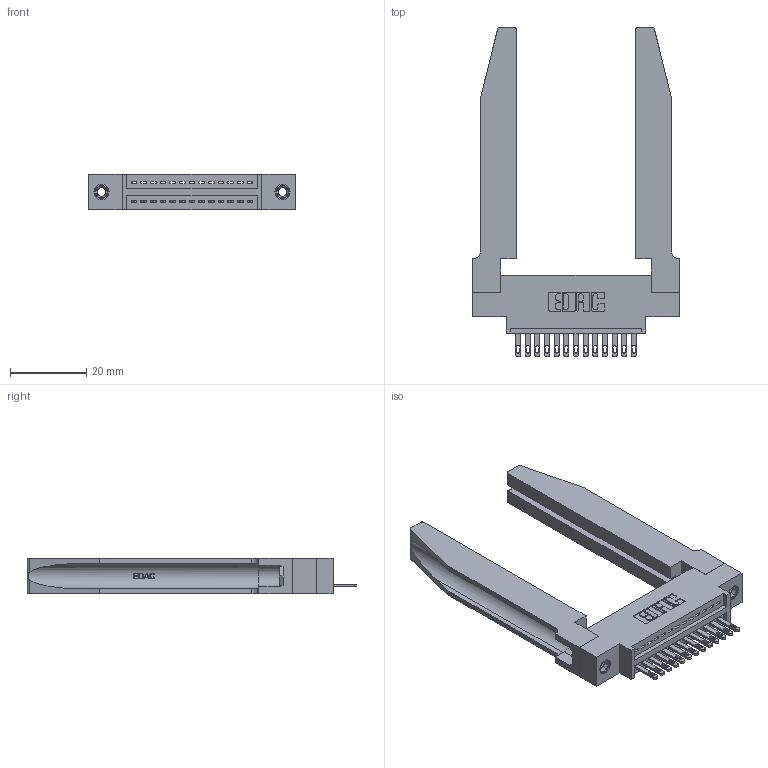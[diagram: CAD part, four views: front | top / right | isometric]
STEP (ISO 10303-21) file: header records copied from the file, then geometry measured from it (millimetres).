
FILE_DESCRIPTION (( 'STEP AP203' ), '1' );
FILE_NAME ('345-013-500-678.STEP', '2019-10-04T02:57:16', ( '' ), ( '' ), 'SwSTEP 2.0', 'SolidWorks 2016', '' );
FILE_SCHEMA (( 'CONFIG_CONTROL_DESIGN' ));
Length unit declared in the file: inch
Products named in the file (5): 345-292-001_345-293-100; 345-250-001_345-250-001-102; 345-220-078_345-220-078; 345 Part_0.170 Offset - 0.156 Dia-TH; 345-013-500-678
Assembly tree (18 placements, depth 2):
  345-013-500-678
    345 Part_0.170 Offset - 0.156 Dia-TH
    345-292-001_345-293-100  x13
    345-250-001_345-250-001-102  x2
    345-220-078_345-220-078  x2
Bounding box: 54.25 x 86.79 x 9.4 mm (x, y, z)
Volume: 12580.7 mm3; surface area: 12999.6 mm2
Topology: 18 solids, 18 shells, 1066 faces, 3145 edges, 2086 vertices
Faces by surface type: plane 668, cylinder 346, bspline 36, cone 12, torus 4
Entity records: 18490 total; most frequent: CARTESIAN_POINT 4102, ORIENTED_EDGE 2946, DIRECTION 2633, EDGE_CURVE 1473, VECTOR 1191, LINE 1191, VERTEX_POINT 976, AXIS2_PLACEMENT_3D 721
